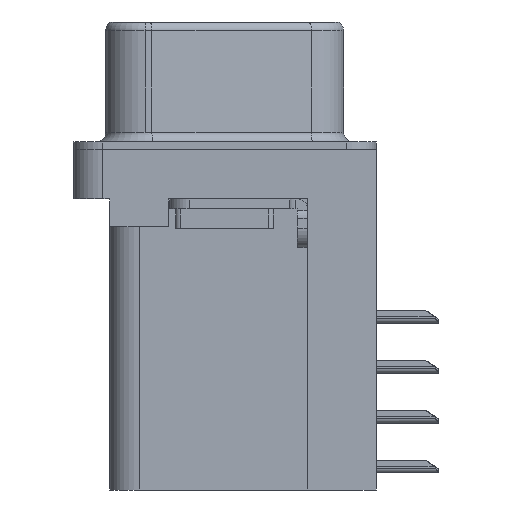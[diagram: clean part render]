
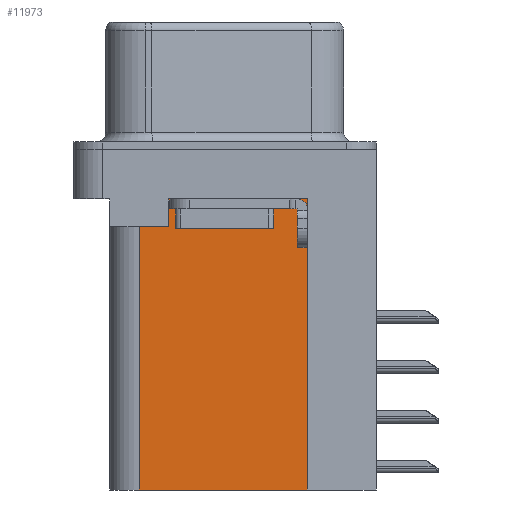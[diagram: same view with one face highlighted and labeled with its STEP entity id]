
A CAD part, left-side view. The second image highlights one B-rep face of the part: STEP entity #11973.
In plain terms, the highlighted planar face has unit normal (-1, 0, 0).
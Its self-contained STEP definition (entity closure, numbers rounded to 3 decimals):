
#974 = CARTESIAN_POINT ( 'NONE',  ( 3.75, 2.85, -2.5 ) ) ;
#2966 = CARTESIAN_POINT ( 'NONE',  ( 3.75, -4.2, -2.5 ) ) ;
#4042 = VERTEX_POINT ( 'NONE', #6405 ) ;
#4075 = VECTOR ( 'NONE', #37346, 1000. ) ;
#4623 = DIRECTION ( 'NONE',  ( 0., 0., 1. ) ) ;
#4842 = CARTESIAN_POINT ( 'NONE',  ( 3.75, -4.2, -17.3 ) ) ;
#6334 = EDGE_LOOP ( 'NONE', ( #20774, #15007, #14015, #15830, #39708, #12228 ) ) ;
#6405 = CARTESIAN_POINT ( 'NONE',  ( 3.75, 4.35, -3.9 ) ) ;
#6857 = DIRECTION ( 'NONE',  ( 0., 0., -1. ) ) ;
#7029 = EDGE_CURVE ( 'NONE', #39696, #4042, #17370, .T. ) ;
#7381 = VERTEX_POINT ( 'NONE', #2966 ) ;
#7834 = CARTESIAN_POINT ( 'NONE',  ( 3.75, -4.2, -17.3 ) ) ;
#8067 = DIRECTION ( 'NONE',  ( 1., 0., 0. ) ) ;
#8607 = CARTESIAN_POINT ( 'NONE',  ( 3.75, 2.85, -3.9 ) ) ;
#10028 = VECTOR ( 'NONE', #38971, 1000. ) ;
#10836 = CARTESIAN_POINT ( 'NONE',  ( 3.75, -4.2, -17.3 ) ) ;
#11973 = ADVANCED_FACE ( 'NONE', ( #33540 ), #23848, .F. ) ;
#12228 = ORIENTED_EDGE ( 'NONE', *, *, #28526, .T. ) ;
#12535 = LINE ( 'NONE', #34080, #4075 ) ;
#12600 = LINE ( 'NONE', #19456, #28479 ) ;
#12868 = AXIS2_PLACEMENT_3D ( 'NONE', #4842, #8067, #30199 ) ;
#13948 = DIRECTION ( 'NONE',  ( 0., 1., 0. ) ) ;
#14015 = ORIENTED_EDGE ( 'NONE', *, *, #39851, .T. ) ;
#15007 = ORIENTED_EDGE ( 'NONE', *, *, #34544, .T. ) ;
#15363 = LINE ( 'NONE', #7834, #39836 ) ;
#15512 = LINE ( 'NONE', #10836, #31431 ) ;
#15830 = ORIENTED_EDGE ( 'NONE', *, *, #7029, .F. ) ;
#16400 = CARTESIAN_POINT ( 'NONE',  ( 3.75, -4.2, -17.3 ) ) ;
#17370 = LINE ( 'NONE', #32468, #10028 ) ;
#19456 = CARTESIAN_POINT ( 'NONE',  ( 3.75, 2.85, -3.9 ) ) ;
#20774 = ORIENTED_EDGE ( 'NONE', *, *, #32568, .T. ) ;
#21096 = LINE ( 'NONE', #27853, #37125 ) ;
#23848 = PLANE ( 'NONE',  #12868 ) ;
#27853 = CARTESIAN_POINT ( 'NONE',  ( 3.75, -4.2, -2.5 ) ) ;
#27997 = VERTEX_POINT ( 'NONE', #974 ) ;
#28479 = VECTOR ( 'NONE', #6857, 1000. ) ;
#28526 = EDGE_CURVE ( 'NONE', #38015, #7381, #15363, .T. ) ;
#30199 = DIRECTION ( 'NONE',  ( 0., 1., 0. ) ) ;
#31208 = VERTEX_POINT ( 'NONE', #8607 ) ;
#31431 = VECTOR ( 'NONE', #13948, 1000. ) ;
#31432 = CARTESIAN_POINT ( 'NONE',  ( 3.75, 4.35, -17.3 ) ) ;
#32468 = CARTESIAN_POINT ( 'NONE',  ( 3.75, 4.35, -17.3 ) ) ;
#32568 = EDGE_CURVE ( 'NONE', #7381, #27997, #21096, .T. ) ;
#33540 = FACE_OUTER_BOUND ( 'NONE', #6334, .T. ) ;
#34080 = CARTESIAN_POINT ( 'NONE',  ( 3.75, 0., -3.9 ) ) ;
#34544 = EDGE_CURVE ( 'NONE', #27997, #31208, #12600, .T. ) ;
#37125 = VECTOR ( 'NONE', #37530, 1000. ) ;
#37346 = DIRECTION ( 'NONE',  ( 0., 1., 0. ) ) ;
#37530 = DIRECTION ( 'NONE',  ( 0., 1., 0. ) ) ;
#38015 = VERTEX_POINT ( 'NONE', #16400 ) ;
#38971 = DIRECTION ( 'NONE',  ( 0., 0., 1. ) ) ;
#39290 = EDGE_CURVE ( 'NONE', #38015, #39696, #15512, .T. ) ;
#39696 = VERTEX_POINT ( 'NONE', #31432 ) ;
#39708 = ORIENTED_EDGE ( 'NONE', *, *, #39290, .F. ) ;
#39836 = VECTOR ( 'NONE', #4623, 1000. ) ;
#39851 = EDGE_CURVE ( 'NONE', #31208, #4042, #12535, .T. ) ;
